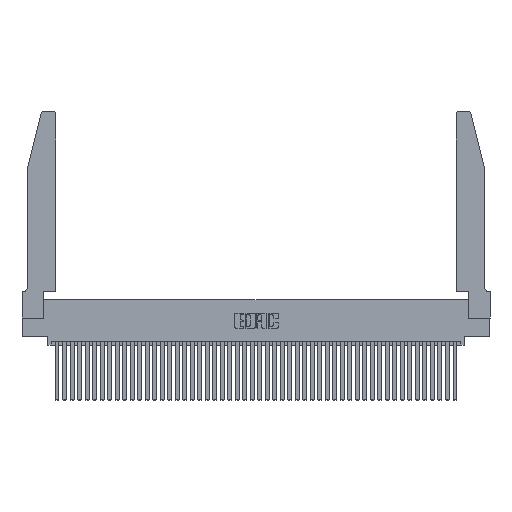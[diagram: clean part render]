
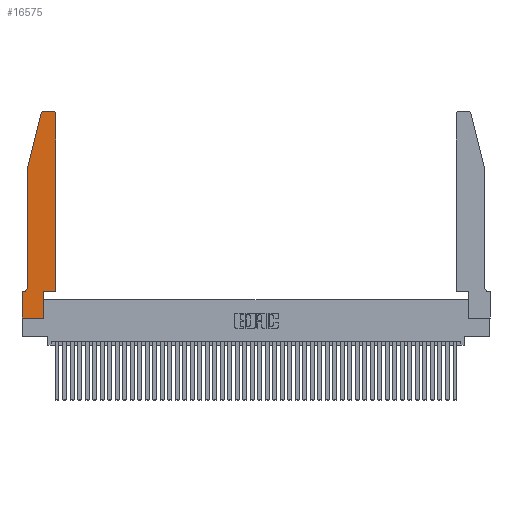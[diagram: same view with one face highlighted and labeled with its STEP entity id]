
A CAD part, top view. The second image highlights one B-rep face of the part: STEP entity #16575.
In plain terms, the highlighted planar face has unit normal (0, 0, 1).
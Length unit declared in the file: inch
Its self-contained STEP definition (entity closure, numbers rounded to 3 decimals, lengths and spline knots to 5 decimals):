
#74 = DIRECTION ( 'NONE',  ( 1., 0., 0. ) ) ;
#235 = VECTOR ( 'NONE', #21578, 39.37008 ) ;
#1034 = AXIS2_PLACEMENT_3D ( 'NONE', #14527, #31415, #74 ) ;
#1095 = DIRECTION ( 'NONE',  ( 0., 1., 0. ) ) ;
#1793 = DIRECTION ( 'NONE',  ( 1., 0., 0. ) ) ;
#2100 = DIRECTION ( 'NONE',  ( 0., -1., 0. ) ) ;
#3089 = CARTESIAN_POINT ( 'NONE',  ( 0.2865, 0., 0.37 ) ) ;
#3169 = DIRECTION ( 'NONE',  ( -1., 0., 0. ) ) ;
#3265 = CARTESIAN_POINT ( 'NONE',  ( 0.4205, 2.72, 0.37 ) ) ;
#3367 = ORIENTED_EDGE ( 'NONE', *, *, #37049, .T. ) ;
#3484 = VERTEX_POINT ( 'NONE', #15828 ) ;
#4328 = ORIENTED_EDGE ( 'NONE', *, *, #25283, .T. ) ;
#4439 = VERTEX_POINT ( 'NONE', #15472 ) ;
#4983 = CIRCLE ( 'NONE', #32004, 0.07 ) ;
#5799 = LINE ( 'NONE', #26724, #31138 ) ;
#6031 = LINE ( 'NONE', #35268, #29706 ) ;
#6647 = VERTEX_POINT ( 'NONE', #25032 ) ;
#7360 = CARTESIAN_POINT ( 'NONE',  ( 0.4505, 0.35, 0.37 ) ) ;
#7521 = CARTESIAN_POINT ( 'NONE',  ( 0., 0.35, 0.37 ) ) ;
#8095 = LINE ( 'NONE', #23676, #35024 ) ;
#8627 = CARTESIAN_POINT ( 'NONE',  ( 0.0755, 2., 0.37 ) ) ;
#9230 = VERTEX_POINT ( 'NONE', #7521 ) ;
#9896 = VERTEX_POINT ( 'NONE', #22027 ) ;
#12101 = CARTESIAN_POINT ( 'NONE',  ( 0.4505, 0.35, 0.37 ) ) ;
#12814 = VECTOR ( 'NONE', #41216, 39.37008 ) ;
#13335 = LINE ( 'NONE', #12101, #41875 ) ;
#13527 = DIRECTION ( 'NONE',  ( -0.239, -0.971, 0. ) ) ;
#13781 = FACE_OUTER_BOUND ( 'NONE', #29170, .T. ) ;
#13910 = DIRECTION ( 'NONE',  ( 0., 0., 1. ) ) ;
#14233 = VERTEX_POINT ( 'NONE', #28240 ) ;
#14442 = LINE ( 'NONE', #8627, #14961 ) ;
#14473 = ORIENTED_EDGE ( 'NONE', *, *, #30661, .T. ) ;
#14527 = CARTESIAN_POINT ( 'NONE',  ( 0.284, 2.72, 0.37 ) ) ;
#14961 = VECTOR ( 'NONE', #13527, 39.37008 ) ;
#15472 = CARTESIAN_POINT ( 'NONE',  ( 0.2865, 0.35, 0.37 ) ) ;
#15635 = VERTEX_POINT ( 'NONE', #36084 ) ;
#15828 = CARTESIAN_POINT ( 'NONE',  ( 0.284, 2.75, 0.37 ) ) ;
#15920 = EDGE_CURVE ( 'NONE', #15635, #32709, #19448, .T. ) ;
#16575 = ADVANCED_FACE ( 'NONE', ( #13781 ), #27728, .T. ) ;
#16706 = ORIENTED_EDGE ( 'NONE', *, *, #35628, .T. ) ;
#16880 = EDGE_CURVE ( 'NONE', #32838, #9230, #6031, .T. ) ;
#16944 = DIRECTION ( 'NONE',  ( 1., 0., 0. ) ) ;
#16968 = ORIENTED_EDGE ( 'NONE', *, *, #16880, .T. ) ;
#18243 = CARTESIAN_POINT ( 'NONE',  ( 0., 0.35, 0.37 ) ) ;
#19185 = ORIENTED_EDGE ( 'NONE', *, *, #25098, .T. ) ;
#19216 = CARTESIAN_POINT ( 'NONE',  ( 0.25487, 2.72718, 0.37 ) ) ;
#19448 = CIRCLE ( 'NONE', #22649, 0.03 ) ;
#19772 = ORIENTED_EDGE ( 'NONE', *, *, #41535, .T. ) ;
#20496 = VECTOR ( 'NONE', #31836, 39.37008 ) ;
#20757 = CIRCLE ( 'NONE', #1034, 0.03 ) ;
#21182 = VERTEX_POINT ( 'NONE', #43887 ) ;
#21578 = DIRECTION ( 'NONE',  ( 0., 1., 0. ) ) ;
#22027 = CARTESIAN_POINT ( 'NONE',  ( 0.0755, 2., 0.37 ) ) ;
#22649 = AXIS2_PLACEMENT_3D ( 'NONE', #3265, #13910, #29119 ) ;
#22712 = DIRECTION ( 'NONE',  ( 0., 0., 1. ) ) ;
#23676 = CARTESIAN_POINT ( 'NONE',  ( 0., 0., 0.37 ) ) ;
#24011 = LINE ( 'NONE', #25550, #33824 ) ;
#25032 = CARTESIAN_POINT ( 'NONE',  ( 0., 0., 0.37 ) ) ;
#25098 = EDGE_CURVE ( 'NONE', #9230, #6647, #8095, .T. ) ;
#25283 = EDGE_CURVE ( 'NONE', #3484, #26849, #20757, .T. ) ;
#25550 = CARTESIAN_POINT ( 'NONE',  ( 0.2865, 0.35, 0.37 ) ) ;
#25687 = CARTESIAN_POINT ( 'NONE',  ( 0.0055, 0.35, 0.37 ) ) ;
#26136 = EDGE_CURVE ( 'NONE', #38511, #4439, #24011, .T. ) ;
#26724 = CARTESIAN_POINT ( 'NONE',  ( 0.0755, 2., 0.37 ) ) ;
#26849 = VERTEX_POINT ( 'NONE', #19216 ) ;
#27728 = PLANE ( 'NONE',  #40784 ) ;
#28077 = DIRECTION ( 'NONE',  ( -1., 0., 0. ) ) ;
#28145 = ORIENTED_EDGE ( 'NONE', *, *, #44206, .T. ) ;
#28214 = LINE ( 'NONE', #44884, #12814 ) ;
#28240 = CARTESIAN_POINT ( 'NONE',  ( 0.0755, 0.42, 0.37 ) ) ;
#29119 = DIRECTION ( 'NONE',  ( 1., 0., 0. ) ) ;
#29170 = EDGE_LOOP ( 'NONE', ( #35931, #4328, #14473, #19772, #3367, #16968, #19185, #28145, #42102, #16706, #31856, #29246 ) ) ;
#29246 = ORIENTED_EDGE ( 'NONE', *, *, #15920, .T. ) ;
#29706 = VECTOR ( 'NONE', #28077, 39.37008 ) ;
#30661 = EDGE_CURVE ( 'NONE', #26849, #9896, #14442, .T. ) ;
#31138 = VECTOR ( 'NONE', #2100, 39.37008 ) ;
#31415 = DIRECTION ( 'NONE',  ( 0., 0., 1. ) ) ;
#31503 = CARTESIAN_POINT ( 'NONE',  ( 0.4205, 2.75, 0.37 ) ) ;
#31836 = DIRECTION ( 'NONE',  ( -1., 0., 0. ) ) ;
#31856 = ORIENTED_EDGE ( 'NONE', *, *, #39120, .T. ) ;
#32004 = AXIS2_PLACEMENT_3D ( 'NONE', #44971, #37908, #3169 ) ;
#32709 = VERTEX_POINT ( 'NONE', #31503 ) ;
#32838 = VERTEX_POINT ( 'NONE', #25687 ) ;
#33824 = VECTOR ( 'NONE', #1095, 39.37008 ) ;
#34892 = CARTESIAN_POINT ( 'NONE',  ( 0.2605, 2.75, 0.37 ) ) ;
#35024 = VECTOR ( 'NONE', #40964, 39.37008 ) ;
#35268 = CARTESIAN_POINT ( 'NONE',  ( 0.0755, 0.35, 0.37 ) ) ;
#35628 = EDGE_CURVE ( 'NONE', #4439, #21182, #13335, .T. ) ;
#35830 = LINE ( 'NONE', #34892, #20496 ) ;
#35931 = ORIENTED_EDGE ( 'NONE', *, *, #36645, .T. ) ;
#36084 = CARTESIAN_POINT ( 'NONE',  ( 0.4505, 2.72, 0.37 ) ) ;
#36645 = EDGE_CURVE ( 'NONE', #32709, #3484, #35830, .T. ) ;
#37049 = EDGE_CURVE ( 'NONE', #14233, #32838, #4983, .T. ) ;
#37908 = DIRECTION ( 'NONE',  ( 0., 0., -1. ) ) ;
#38511 = VERTEX_POINT ( 'NONE', #3089 ) ;
#39120 = EDGE_CURVE ( 'NONE', #21182, #15635, #44155, .T. ) ;
#40784 = AXIS2_PLACEMENT_3D ( 'NONE', #18243, #22712, #16944 ) ;
#40964 = DIRECTION ( 'NONE',  ( 0., -1., 0. ) ) ;
#41216 = DIRECTION ( 'NONE',  ( 1., 0., 0. ) ) ;
#41535 = EDGE_CURVE ( 'NONE', #9896, #14233, #5799, .T. ) ;
#41875 = VECTOR ( 'NONE', #1793, 39.37008 ) ;
#42102 = ORIENTED_EDGE ( 'NONE', *, *, #26136, .T. ) ;
#43887 = CARTESIAN_POINT ( 'NONE',  ( 0.4505, 0.35, 0.37 ) ) ;
#44155 = LINE ( 'NONE', #7360, #235 ) ;
#44206 = EDGE_CURVE ( 'NONE', #6647, #38511, #28214, .T. ) ;
#44884 = CARTESIAN_POINT ( 'NONE',  ( 0., 0., 0.37 ) ) ;
#44971 = CARTESIAN_POINT ( 'NONE',  ( 0.0055, 0.42, 0.37 ) ) ;
